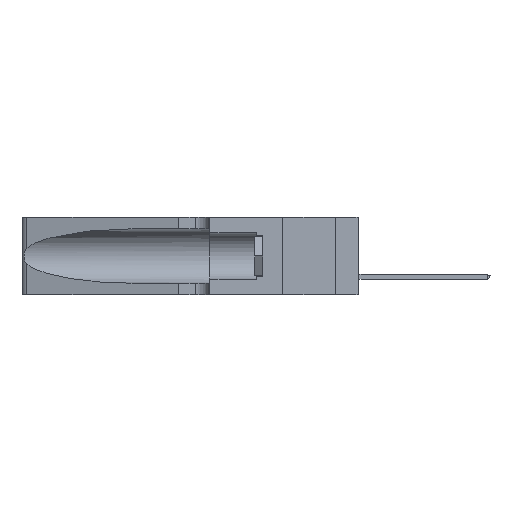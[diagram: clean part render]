
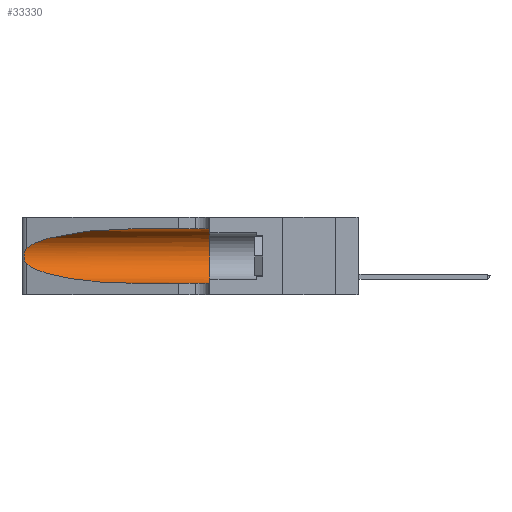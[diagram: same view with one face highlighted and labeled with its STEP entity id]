
A CAD part, left-side view. The second image highlights one B-rep face of the part: STEP entity #33330.
In plain terms, the highlighted cylindrical face has radius 3.308 mm (diameter 6.617 mm), a partial arc.
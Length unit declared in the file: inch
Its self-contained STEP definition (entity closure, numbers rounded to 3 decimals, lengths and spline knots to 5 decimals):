
#591 = DIRECTION ( 'NONE',  ( 0., -1., 0. ) ) ;
#2174 = EDGE_CURVE ( 'NONE', #33391, #35764, #20223, .T. ) ;
#3046 = CARTESIAN_POINT ( 'NONE',  ( 0.1305, 1.61858, 0.185 ) ) ;
#4865 = ORIENTED_EDGE ( 'NONE', *, *, #2174, .T. ) ;
#4930 = CARTESIAN_POINT ( 'NONE',  ( 0.25487, 1.22718, 0.14631 ) ) ;
#5558 = CARTESIAN_POINT ( 'NONE',  ( 0.26075, 1.23896, 0.19203 ) ) ;
#5677 = EDGE_CURVE ( 'NONE', #10570, #20597, #29026, .T. ) ;
#5695 = ORIENTED_EDGE ( 'NONE', *, *, #11403, .T. ) ;
#5910 = CARTESIAN_POINT ( 'NONE',  ( 0.25854, 1.2359, 0.20912 ) ) ;
#5928 = EDGE_CURVE ( 'NONE', #23890, #20597, #35370, .T. ) ;
#6900 = VECTOR ( 'NONE', #591, 39.37008 ) ;
#7061 = CARTESIAN_POINT ( 'NONE',  ( 0.2373, 1.15595, 0.08982 ) ) ;
#7065 = AXIS2_PLACEMENT_3D ( 'NONE', #3046, #12888, #36447 ) ;
#8457 = CARTESIAN_POINT ( 'NONE',  ( 0.25639, 1.23186, 0.15144 ) ) ;
#9513 =( BOUNDED_CURVE ( )  B_SPLINE_CURVE ( 3, ( #13037, #25447, #30479, #10899 ),
 .UNSPECIFIED., .F., .T. ) 
 B_SPLINE_CURVE_WITH_KNOTS ( ( 4, 4 ),
 ( 1.5708, 2.84003 ),
 .UNSPECIFIED. ) 
 CURVE ( )  GEOMETRIC_REPRESENTATION_ITEM ( )  RATIONAL_B_SPLINE_CURVE ( ( 1., 0.87, 0.87, 1. ) ) 
 REPRESENTATION_ITEM ( '' )  );
#10570 = VERTEX_POINT ( 'NONE', #24253 ) ;
#10899 = CARTESIAN_POINT ( 'NONE',  ( 0.25487, 1.22718, 0.22369 ) ) ;
#11046 = AXIS2_PLACEMENT_3D ( 'NONE', #26129, #29011, #29485 ) ;
#11403 = EDGE_CURVE ( 'NONE', #32632, #33391, #9513, .T. ) ;
#12888 = DIRECTION ( 'NONE',  ( 0., -1., 0. ) ) ;
#13037 = CARTESIAN_POINT ( 'NONE',  ( 0.1305, 0.72297, 0.31525 ) ) ;
#13137 = CARTESIAN_POINT ( 'NONE',  ( 0.25487, 1.22718, 0.14631 ) ) ;
#13546 = VECTOR ( 'NONE', #17846, 39.37008 ) ;
#14078 = ORIENTED_EDGE ( 'NONE', *, *, #5677, .T. ) ;
#14760 = CARTESIAN_POINT ( 'NONE',  ( 0.25639, 1.23184, 0.21858 ) ) ;
#15637 = CARTESIAN_POINT ( 'NONE',  ( 0.25487, 1.22718, 0.22369 ) ) ;
#15702 = ORIENTED_EDGE ( 'NONE', *, *, #15934, .F. ) ;
#15932 = CARTESIAN_POINT ( 'NONE',  ( 0.1305, 0.72297, 0.05475 ) ) ;
#15934 = EDGE_CURVE ( 'NONE', #32632, #23890, #28321, .T. ) ;
#17331 = EDGE_LOOP ( 'NONE', ( #5695, #4865, #27566, #14078, #33238, #15702 ) ) ;
#17846 = DIRECTION ( 'NONE',  ( 0., -1., 0. ) ) ;
#18406 = CARTESIAN_POINT ( 'NONE',  ( 0.1305, 1.61858, 0.31525 ) ) ;
#19190 = CARTESIAN_POINT ( 'NONE',  ( 0.1305, 0.35, 0.05475 ) ) ;
#20223 = B_SPLINE_CURVE_WITH_KNOTS ( 'NONE', 3,
 ( #32183, #23402, #14760, #35137, #5910, #22912, #5558, #34654, #23028, #25901, #29029, #8457, #28796, #34785 ),
 .UNSPECIFIED., .F., .F.,
 ( 4, 2, 2, 2, 2, 2, 4 ),
 ( 0., 0.00027, 0.00053, 0.00107, 0.0016, 0.00187, 0.00214 ),
 .UNSPECIFIED. ) ;
#20597 = VERTEX_POINT ( 'NONE', #19190 ) ;
#21623 = EDGE_CURVE ( 'NONE', #35764, #10570, #30954, .T. ) ;
#22510 = FACE_OUTER_BOUND ( 'NONE', #17331, .T. ) ;
#22912 = CARTESIAN_POINT ( 'NONE',  ( 0.26018, 1.23835, 0.19895 ) ) ;
#23028 = CARTESIAN_POINT ( 'NONE',  ( 0.26017, 1.23833, 0.17102 ) ) ;
#23402 = CARTESIAN_POINT ( 'NONE',  ( 0.25555, 1.22994, 0.2215 ) ) ;
#23890 = VERTEX_POINT ( 'NONE', #32706 ) ;
#24253 = CARTESIAN_POINT ( 'NONE',  ( 0.1305, 0.72297, 0.05475 ) ) ;
#24296 = CARTESIAN_POINT ( 'NONE',  ( 0.1305, 1.61858, 0.05475 ) ) ;
#25447 = CARTESIAN_POINT ( 'NONE',  ( 0.18966, 0.96281, 0.31525 ) ) ;
#25901 = CARTESIAN_POINT ( 'NONE',  ( 0.25856, 1.23593, 0.16098 ) ) ;
#26129 = CARTESIAN_POINT ( 'NONE',  ( 0.1305, 0.35, 0.185 ) ) ;
#27566 = ORIENTED_EDGE ( 'NONE', *, *, #21623, .T. ) ;
#28321 = LINE ( 'NONE', #18406, #6900 ) ;
#28796 = CARTESIAN_POINT ( 'NONE',  ( 0.25555, 1.22993, 0.14849 ) ) ;
#29011 = DIRECTION ( 'NONE',  ( 0., 1., 0. ) ) ;
#29026 = LINE ( 'NONE', #24296, #13546 ) ;
#29029 = CARTESIAN_POINT ( 'NONE',  ( 0.25789, 1.23486, 0.15765 ) ) ;
#29485 = DIRECTION ( 'NONE',  ( 0., 0., 1. ) ) ;
#30379 = CARTESIAN_POINT ( 'NONE',  ( 0.1305, 0.72297, 0.31525 ) ) ;
#30479 = CARTESIAN_POINT ( 'NONE',  ( 0.2373, 1.15595, 0.28018 ) ) ;
#30954 =( BOUNDED_CURVE ( )  B_SPLINE_CURVE ( 3, ( #13137, #7061, #33387, #15932 ),
 .UNSPECIFIED., .F., .F. ) 
 B_SPLINE_CURVE_WITH_KNOTS ( ( 4, 4 ),
 ( 3.44316, 4.71239 ),
 .UNSPECIFIED. ) 
 CURVE ( )  GEOMETRIC_REPRESENTATION_ITEM ( )  RATIONAL_B_SPLINE_CURVE ( ( 1., 0.87, 0.87, 1. ) ) 
 REPRESENTATION_ITEM ( '' )  );
#32183 = CARTESIAN_POINT ( 'NONE',  ( 0.25487, 1.22718, 0.22369 ) ) ;
#32632 = VERTEX_POINT ( 'NONE', #30379 ) ;
#32706 = CARTESIAN_POINT ( 'NONE',  ( 0.1305, 0.35, 0.31525 ) ) ;
#33238 = ORIENTED_EDGE ( 'NONE', *, *, #5928, .F. ) ;
#33330 = ADVANCED_FACE ( 'NONE', ( #22510 ), #36174, .F. ) ;
#33387 = CARTESIAN_POINT ( 'NONE',  ( 0.18966, 0.96281, 0.05475 ) ) ;
#33391 = VERTEX_POINT ( 'NONE', #15637 ) ;
#34654 = CARTESIAN_POINT ( 'NONE',  ( 0.26075, 1.23896, 0.178 ) ) ;
#34785 = CARTESIAN_POINT ( 'NONE',  ( 0.25487, 1.22718, 0.14631 ) ) ;
#35137 = CARTESIAN_POINT ( 'NONE',  ( 0.25787, 1.23484, 0.2124 ) ) ;
#35370 = CIRCLE ( 'NONE', #11046, 0.13025 ) ;
#35764 = VERTEX_POINT ( 'NONE', #4930 ) ;
#36174 = CYLINDRICAL_SURFACE ( 'NONE', #7065, 0.13025 ) ;
#36447 = DIRECTION ( 'NONE',  ( 0., 0., -1. ) ) ;
